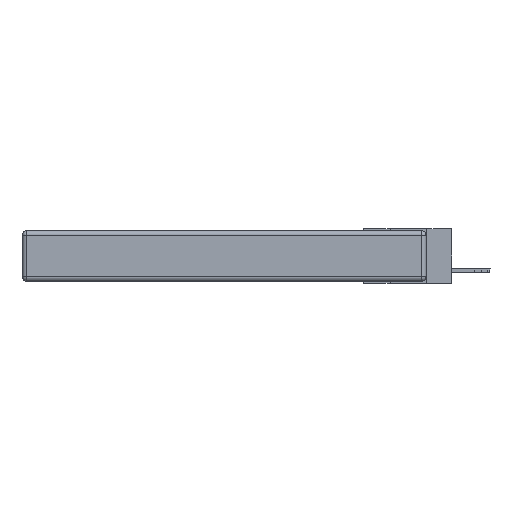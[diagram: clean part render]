
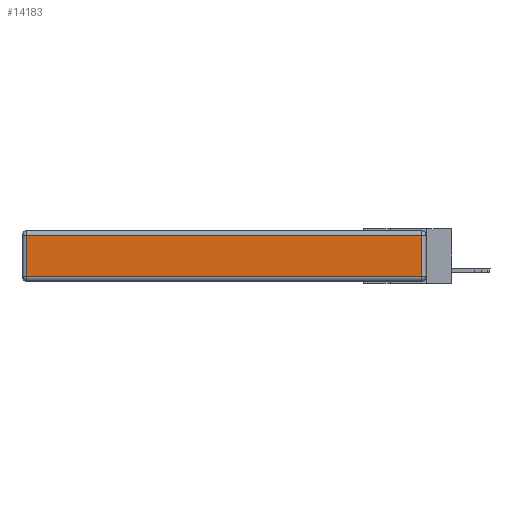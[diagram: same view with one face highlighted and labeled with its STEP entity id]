
A CAD part, left-side view. The second image highlights one B-rep face of the part: STEP entity #14183.
In plain terms, the highlighted planar face has unit normal (-1, 0, 0).
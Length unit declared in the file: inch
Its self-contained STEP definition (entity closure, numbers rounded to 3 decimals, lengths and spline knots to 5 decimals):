
#337 = ORIENTED_EDGE ( 'NONE', *, *, #18377, .T. ) ;
#702 = EDGE_CURVE ( 'NONE', #1607, #7515, #16726, .T. ) ;
#762 = FACE_OUTER_BOUND ( 'NONE', #15688, .T. ) ;
#854 = CARTESIAN_POINT ( 'NONE',  ( 0., 2.72, -0.343 ) ) ;
#1121 = VERTEX_POINT ( 'NONE', #14757 ) ;
#1607 = VERTEX_POINT ( 'NONE', #2809 ) ;
#2176 = EDGE_CURVE ( 'NONE', #1121, #1607, #7693, .T. ) ;
#2665 = ORIENTED_EDGE ( 'NONE', *, *, #702, .T. ) ;
#2809 = CARTESIAN_POINT ( 'NONE',  ( 0., 2.72, -0.313 ) ) ;
#3925 = DIRECTION ( 'NONE',  ( 0., -1., 0. ) ) ;
#4101 = CARTESIAN_POINT ( 'NONE',  ( 0., 0., -0.313 ) ) ;
#5139 = VECTOR ( 'NONE', #17577, 39.37008 ) ;
#5311 = LINE ( 'NONE', #13097, #8688 ) ;
#5420 = VECTOR ( 'NONE', #18087, 39.37008 ) ;
#6070 = ORIENTED_EDGE ( 'NONE', *, *, #14710, .T. ) ;
#6307 = DIRECTION ( 'NONE',  ( 0., 0., 1. ) ) ;
#7514 = CARTESIAN_POINT ( 'NONE',  ( 0., 0.03, -0.313 ) ) ;
#7515 = VERTEX_POINT ( 'NONE', #7514 ) ;
#7573 = PLANE ( 'NONE',  #8392 ) ;
#7625 = CARTESIAN_POINT ( 'NONE',  ( 0., 0.03, -0.343 ) ) ;
#7693 = LINE ( 'NONE', #854, #5420 ) ;
#8392 = AXIS2_PLACEMENT_3D ( 'NONE', #11962, #9148, #6307 ) ;
#8688 = VECTOR ( 'NONE', #14716, 39.37008 ) ;
#9148 = DIRECTION ( 'NONE',  ( -1., 0., 0. ) ) ;
#10329 = VERTEX_POINT ( 'NONE', #18202 ) ;
#10735 = LINE ( 'NONE', #7625, #5139 ) ;
#11962 = CARTESIAN_POINT ( 'NONE',  ( 0., 0., -0.343 ) ) ;
#13097 = CARTESIAN_POINT ( 'NONE',  ( 0., 2.75, -0.03 ) ) ;
#14183 = ADVANCED_FACE ( 'NONE', ( #762 ), #7573, .T. ) ;
#14710 = EDGE_CURVE ( 'NONE', #10329, #1121, #5311, .T. ) ;
#14716 = DIRECTION ( 'NONE',  ( 0., 1., 0. ) ) ;
#14757 = CARTESIAN_POINT ( 'NONE',  ( 0., 2.72, -0.03 ) ) ;
#15688 = EDGE_LOOP ( 'NONE', ( #2665, #337, #6070, #18714 ) ) ;
#16039 = VECTOR ( 'NONE', #3925, 39.37008 ) ;
#16726 = LINE ( 'NONE', #4101, #16039 ) ;
#17577 = DIRECTION ( 'NONE',  ( 0., 0., 1. ) ) ;
#18087 = DIRECTION ( 'NONE',  ( 0., 0., -1. ) ) ;
#18202 = CARTESIAN_POINT ( 'NONE',  ( 0., 0.03, -0.03 ) ) ;
#18377 = EDGE_CURVE ( 'NONE', #7515, #10329, #10735, .T. ) ;
#18714 = ORIENTED_EDGE ( 'NONE', *, *, #2176, .T. ) ;
